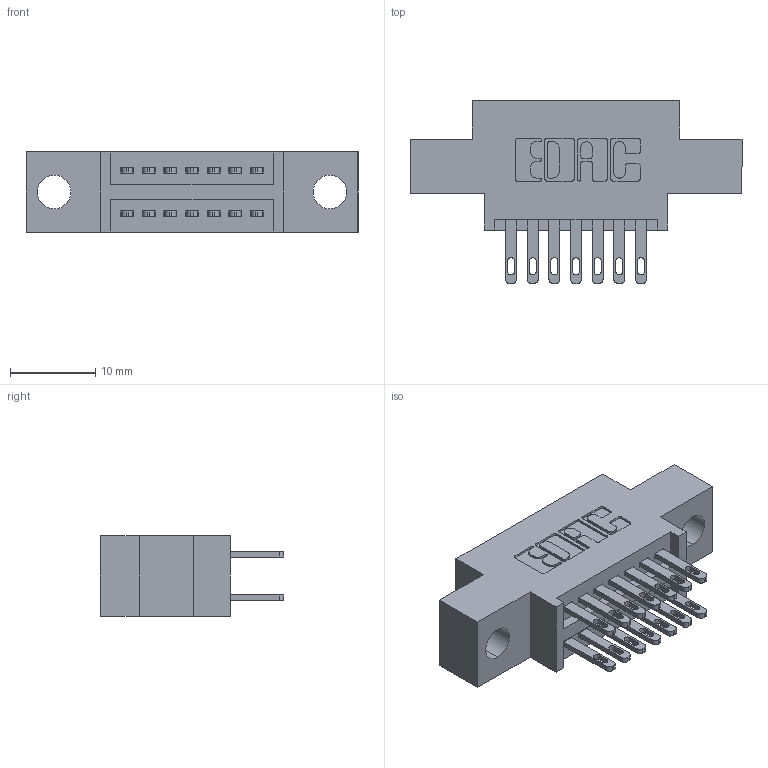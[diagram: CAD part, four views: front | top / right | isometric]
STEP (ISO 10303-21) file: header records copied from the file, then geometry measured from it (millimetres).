
FILE_DESCRIPTION (( 'STEP AP203' ), '1' );
FILE_NAME ('895-014-500-804.STEP', '2020-09-25T03:06:18', ( '' ), ( '' ), 'SwSTEP 2.0', 'SolidWorks 2020', '' );
FILE_SCHEMA (( 'CONFIG_CONTROL_DESIGN' ));
Length unit declared in the file: inch
Products named in the file (3): 895-014-500-804; 845 Part_0.170 Offset - 0.156 Dia-TH; 345-292-001_345-293-100
Assembly tree (15 placements, depth 2):
  895-014-500-804
    845 Part_0.170 Offset - 0.156 Dia-TH
    345-292-001_345-293-100  x14
Bounding box: 38.99 x 21.51 x 9.4 mm (x, y, z)
Volume: 3304.1 mm3; surface area: 4307.6 mm2
Topology: 15 solids, 15 shells, 774 faces, 2327 edges, 1550 vertices
Faces by surface type: plane 462, cylinder 312
Entity records: 10269 total; most frequent: CARTESIAN_POINT 1756, ORIENTED_EDGE 1690, DIRECTION 1593, EDGE_CURVE 845, VECTOR 681, LINE 681, VERTEX_POINT 562, AXIS2_PLACEMENT_3D 456
